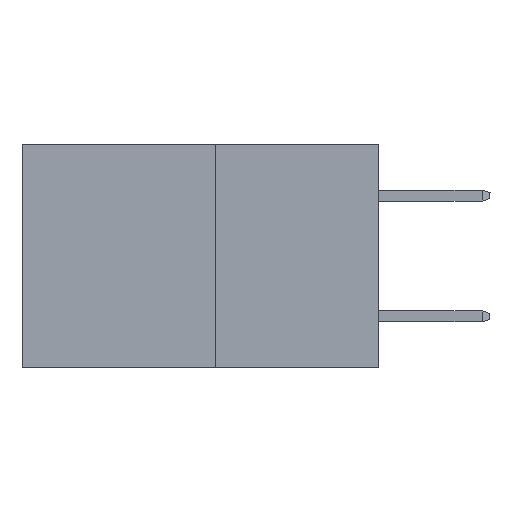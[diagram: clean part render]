
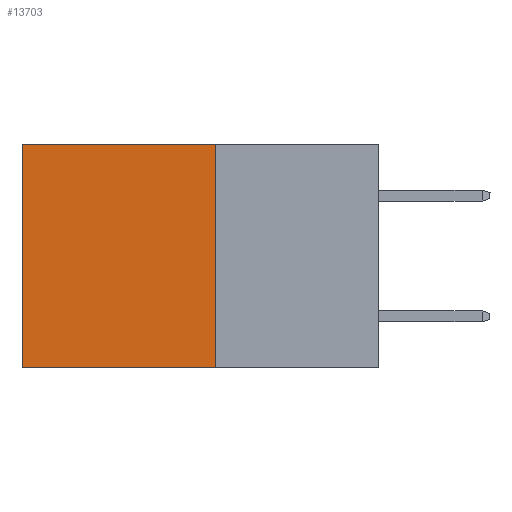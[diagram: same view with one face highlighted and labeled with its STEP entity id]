
A CAD part, left-side view. The second image highlights one B-rep face of the part: STEP entity #13703.
In plain terms, the highlighted planar face has unit normal (-1, 0, 0).
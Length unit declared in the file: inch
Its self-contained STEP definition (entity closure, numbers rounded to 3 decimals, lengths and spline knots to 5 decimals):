
#28 = VECTOR ( 'NONE', #11855, 39.37008 ) ;
#382 = FACE_OUTER_BOUND ( 'NONE', #12079, .T. ) ;
#394 = PLANE ( 'NONE',  #1661 ) ;
#1546 = DIRECTION ( 'NONE',  ( 0., 0., -1. ) ) ;
#1661 = AXIS2_PLACEMENT_3D ( 'NONE', #12972, #8417, #1546 ) ;
#1730 = LINE ( 'NONE', #5840, #10857 ) ;
#3007 = VERTEX_POINT ( 'NONE', #8039 ) ;
#3195 = VERTEX_POINT ( 'NONE', #7233 ) ;
#3787 = CARTESIAN_POINT ( 'NONE',  ( 0.277, 0.59, -0.37 ) ) ;
#3806 = VERTEX_POINT ( 'NONE', #8873 ) ;
#3872 = LINE ( 'NONE', #3787, #9636 ) ;
#4033 = EDGE_CURVE ( 'NONE', #3806, #11253, #4860, .T. ) ;
#4225 = ORIENTED_EDGE ( 'NONE', *, *, #13721, .T. ) ;
#4860 = LINE ( 'NONE', #10343, #10603 ) ;
#5171 = ORIENTED_EDGE ( 'NONE', *, *, #4033, .F. ) ;
#5840 = CARTESIAN_POINT ( 'NONE',  ( 0.277, 0.27, -0.37 ) ) ;
#6113 = LINE ( 'NONE', #10701, #28 ) ;
#7233 = CARTESIAN_POINT ( 'NONE',  ( 0.277, 0.59, 0. ) ) ;
#7553 = ORIENTED_EDGE ( 'NONE', *, *, #9731, .F. ) ;
#7884 = EDGE_CURVE ( 'NONE', #3195, #3007, #3872, .T. ) ;
#8039 = CARTESIAN_POINT ( 'NONE',  ( 0.277, 0.59, -0.37 ) ) ;
#8101 = DIRECTION ( 'NONE',  ( 0., 0., -1. ) ) ;
#8417 = DIRECTION ( 'NONE',  ( 1., 0., 0. ) ) ;
#8873 = CARTESIAN_POINT ( 'NONE',  ( 0.277, 0.27, 0. ) ) ;
#9221 = ORIENTED_EDGE ( 'NONE', *, *, #7884, .T. ) ;
#9636 = VECTOR ( 'NONE', #12977, 39.37008 ) ;
#9731 = EDGE_CURVE ( 'NONE', #11253, #3007, #1730, .T. ) ;
#10343 = CARTESIAN_POINT ( 'NONE',  ( 0.277, 0.27, -0.37 ) ) ;
#10603 = VECTOR ( 'NONE', #8101, 39.37008 ) ;
#10701 = CARTESIAN_POINT ( 'NONE',  ( 0.277, 0.27, 0. ) ) ;
#10857 = VECTOR ( 'NONE', #13855, 39.37008 ) ;
#11253 = VERTEX_POINT ( 'NONE', #11511 ) ;
#11511 = CARTESIAN_POINT ( 'NONE',  ( 0.277, 0.27, -0.37 ) ) ;
#11855 = DIRECTION ( 'NONE',  ( 0., 1., 0. ) ) ;
#12079 = EDGE_LOOP ( 'NONE', ( #9221, #7553, #5171, #4225 ) ) ;
#12972 = CARTESIAN_POINT ( 'NONE',  ( 0.277, 0.27, -0.37 ) ) ;
#12977 = DIRECTION ( 'NONE',  ( 0., 0., -1. ) ) ;
#13703 = ADVANCED_FACE ( 'NONE', ( #382 ), #394, .F. ) ;
#13721 = EDGE_CURVE ( 'NONE', #3806, #3195, #6113, .T. ) ;
#13855 = DIRECTION ( 'NONE',  ( 0., 1., 0. ) ) ;
